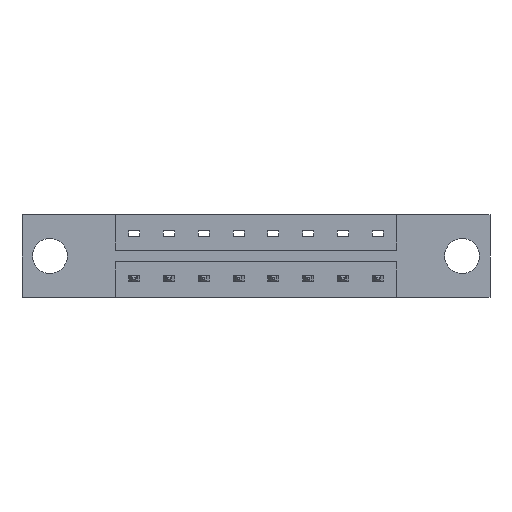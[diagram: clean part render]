
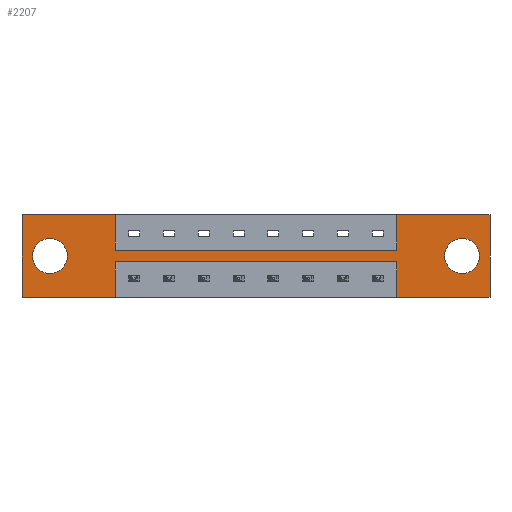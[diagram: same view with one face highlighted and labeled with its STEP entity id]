
A CAD part, front view. The second image highlights one B-rep face of the part: STEP entity #2207.
In plain terms, the highlighted planar face has unit normal (0, -1, 0).
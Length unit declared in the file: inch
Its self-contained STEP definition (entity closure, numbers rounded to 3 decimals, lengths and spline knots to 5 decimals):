
#139 = CARTESIAN_POINT ( 'NONE',  ( 0.125, 0., -0.107 ) ) ;
#160 = DIRECTION ( 'NONE',  ( 0., 1., 0. ) ) ;
#165 = CARTESIAN_POINT ( 'NONE',  ( 1.6785, 0., 0. ) ) ;
#324 = VERTEX_POINT ( 'NONE', #4264 ) ;
#367 = EDGE_CURVE ( 'NONE', #1852, #6719, #958, .T. ) ;
#611 = AXIS2_PLACEMENT_3D ( 'NONE', #2111, #160, #5095 ) ;
#616 = VECTOR ( 'NONE', #8769, 39.37008 ) ;
#666 = AXIS2_PLACEMENT_3D ( 'NONE', #2373, #1766, #8126 ) ;
#777 = CARTESIAN_POINT ( 'NONE',  ( 0., 0., 0. ) ) ;
#881 = ORIENTED_EDGE ( 'NONE', *, *, #7496, .F. ) ;
#884 = ORIENTED_EDGE ( 'NONE', *, *, #993, .F. ) ;
#929 = DIRECTION ( 'NONE',  ( -1., 0., 0. ) ) ;
#958 = LINE ( 'NONE', #1701, #5519 ) ;
#993 = EDGE_CURVE ( 'NONE', #8271, #3532, #1184, .T. ) ;
#1001 = DIRECTION ( 'NONE',  ( 1., 0., 0. ) ) ;
#1050 = CIRCLE ( 'NONE', #7961, 0.078 ) ;
#1163 = DIRECTION ( 'NONE',  ( 0., 0., -1. ) ) ;
#1184 = LINE ( 'NONE', #4027, #3704 ) ;
#1374 = ORIENTED_EDGE ( 'NONE', *, *, #8240, .F. ) ;
#1465 = DIRECTION ( 'NONE',  ( 0., 0., -1. ) ) ;
#1591 = CARTESIAN_POINT ( 'NONE',  ( 0.125, 0., -0.263 ) ) ;
#1646 = CARTESIAN_POINT ( 'NONE',  ( 0.4175, 0., 0. ) ) ;
#1683 = ORIENTED_EDGE ( 'NONE', *, *, #1780, .T. ) ;
#1701 = CARTESIAN_POINT ( 'NONE',  ( 1.6785, 0., -0.1585 ) ) ;
#1766 = DIRECTION ( 'NONE',  ( 0., 1., 0. ) ) ;
#1780 = EDGE_CURVE ( 'NONE', #3923, #2492, #1050, .T. ) ;
#1852 = VERTEX_POINT ( 'NONE', #2657 ) ;
#2101 = VECTOR ( 'NONE', #7195, 39.37008 ) ;
#2111 = CARTESIAN_POINT ( 'NONE',  ( 1.971, 0., -0.185 ) ) ;
#2207 = ADVANCED_FACE ( 'NONE', ( #9029, #5955, #2548 ), #5431, .T. ) ;
#2288 = CARTESIAN_POINT ( 'NONE',  ( 0., 0., 0. ) ) ;
#2294 = DIRECTION ( 'NONE',  ( 0., 0., 1. ) ) ;
#2360 = EDGE_CURVE ( 'NONE', #2492, #3923, #5554, .T. ) ;
#2368 = CARTESIAN_POINT ( 'NONE',  ( 0.125, 0., -0.185 ) ) ;
#2373 = CARTESIAN_POINT ( 'NONE',  ( 0.125, 0., -0.185 ) ) ;
#2471 = CARTESIAN_POINT ( 'NONE',  ( 1.971, 0., -0.185 ) ) ;
#2492 = VERTEX_POINT ( 'NONE', #3578 ) ;
#2548 = FACE_OUTER_BOUND ( 'NONE', #8283, .T. ) ;
#2581 = VECTOR ( 'NONE', #4423, 39.37008 ) ;
#2657 = CARTESIAN_POINT ( 'NONE',  ( 1.6785, 0., -0.1585 ) ) ;
#2668 = CARTESIAN_POINT ( 'NONE',  ( 1.6785, 0., -0.37 ) ) ;
#2714 = ORIENTED_EDGE ( 'NONE', *, *, #3780, .F. ) ;
#2778 = EDGE_CURVE ( 'NONE', #7587, #2853, #3658, .T. ) ;
#2853 = VERTEX_POINT ( 'NONE', #5265 ) ;
#2858 = VERTEX_POINT ( 'NONE', #139 ) ;
#3025 = CIRCLE ( 'NONE', #3169, 0.078 ) ;
#3159 = AXIS2_PLACEMENT_3D ( 'NONE', #8307, #8855, #7776 ) ;
#3169 = AXIS2_PLACEMENT_3D ( 'NONE', #2368, #5251, #8700 ) ;
#3174 = EDGE_CURVE ( 'NONE', #2858, #6212, #3025, .T. ) ;
#3183 = CARTESIAN_POINT ( 'NONE',  ( 0.4175, 0., -0.1585 ) ) ;
#3208 = DIRECTION ( 'NONE',  ( 0., 0., -1. ) ) ;
#3321 = EDGE_CURVE ( 'NONE', #2853, #8271, #4490, .T. ) ;
#3480 = VECTOR ( 'NONE', #1001, 39.37008 ) ;
#3532 = VERTEX_POINT ( 'NONE', #3537 ) ;
#3537 = CARTESIAN_POINT ( 'NONE',  ( 0.4175, 0., -0.1585 ) ) ;
#3578 = CARTESIAN_POINT ( 'NONE',  ( 1.971, 0., -0.107 ) ) ;
#3579 = CARTESIAN_POINT ( 'NONE',  ( 0.4175, 0., -0.2115 ) ) ;
#3658 = LINE ( 'NONE', #2288, #616 ) ;
#3704 = VECTOR ( 'NONE', #3208, 39.37008 ) ;
#3780 = EDGE_CURVE ( 'NONE', #6344, #8059, #5052, .T. ) ;
#3784 = ORIENTED_EDGE ( 'NONE', *, *, #6239, .T. ) ;
#3793 = LINE ( 'NONE', #4643, #6399 ) ;
#3923 = VERTEX_POINT ( 'NONE', #4716 ) ;
#4027 = CARTESIAN_POINT ( 'NONE',  ( 0.4175, 0., -0.1585 ) ) ;
#4037 = ORIENTED_EDGE ( 'NONE', *, *, #8281, .F. ) ;
#4127 = EDGE_CURVE ( 'NONE', #8059, #7587, #8682, .T. ) ;
#4264 = CARTESIAN_POINT ( 'NONE',  ( 1.6785, 0., -0.2115 ) ) ;
#4271 = CARTESIAN_POINT ( 'NONE',  ( 0., 0., -0.37 ) ) ;
#4311 = CARTESIAN_POINT ( 'NONE',  ( 2.096, 0., 0. ) ) ;
#4337 = EDGE_CURVE ( 'NONE', #6719, #4370, #6734, .T. ) ;
#4370 = VERTEX_POINT ( 'NONE', #5368 ) ;
#4417 = LINE ( 'NONE', #7296, #8925 ) ;
#4423 = DIRECTION ( 'NONE',  ( -1., 0., 0. ) ) ;
#4490 = LINE ( 'NONE', #777, #8286 ) ;
#4643 = CARTESIAN_POINT ( 'NONE',  ( 0.4175, 0., -0.2115 ) ) ;
#4656 = ORIENTED_EDGE ( 'NONE', *, *, #2778, .F. ) ;
#4716 = CARTESIAN_POINT ( 'NONE',  ( 1.971, 0., -0.263 ) ) ;
#4785 = ORIENTED_EDGE ( 'NONE', *, *, #7455, .F. ) ;
#5052 = LINE ( 'NONE', #3579, #7989 ) ;
#5095 = DIRECTION ( 'NONE',  ( 0., 0., -1. ) ) ;
#5203 = EDGE_LOOP ( 'NONE', ( #6758, #1683 ) ) ;
#5251 = DIRECTION ( 'NONE',  ( 0., 1., 0. ) ) ;
#5265 = CARTESIAN_POINT ( 'NONE',  ( 0., 0., 0. ) ) ;
#5368 = CARTESIAN_POINT ( 'NONE',  ( 2.096, 0., 0. ) ) ;
#5370 = EDGE_CURVE ( 'NONE', #8772, #8592, #8882, .T. ) ;
#5391 = DIRECTION ( 'NONE',  ( 1., 0., 0. ) ) ;
#5431 = PLANE ( 'NONE',  #3159 ) ;
#5436 = ORIENTED_EDGE ( 'NONE', *, *, #3174, .T. ) ;
#5519 = VECTOR ( 'NONE', #6508, 39.37008 ) ;
#5554 = CIRCLE ( 'NONE', #611, 0.078 ) ;
#5911 = VECTOR ( 'NONE', #8155, 39.37008 ) ;
#5955 = FACE_BOUND ( 'NONE', #8947, .T. ) ;
#5999 = CARTESIAN_POINT ( 'NONE',  ( 0., 0., -0.37 ) ) ;
#6203 = ORIENTED_EDGE ( 'NONE', *, *, #4127, .F. ) ;
#6212 = VERTEX_POINT ( 'NONE', #1591 ) ;
#6239 = EDGE_CURVE ( 'NONE', #6212, #2858, #8642, .T. ) ;
#6275 = CARTESIAN_POINT ( 'NONE',  ( 0.4175, 0., -0.37 ) ) ;
#6344 = VERTEX_POINT ( 'NONE', #7643 ) ;
#6399 = VECTOR ( 'NONE', #929, 39.37008 ) ;
#6508 = DIRECTION ( 'NONE',  ( 0., 0., 1. ) ) ;
#6719 = VERTEX_POINT ( 'NONE', #165 ) ;
#6734 = LINE ( 'NONE', #7398, #3480 ) ;
#6758 = ORIENTED_EDGE ( 'NONE', *, *, #2360, .T. ) ;
#7195 = DIRECTION ( 'NONE',  ( 0., 0., -1. ) ) ;
#7238 = ORIENTED_EDGE ( 'NONE', *, *, #5370, .F. ) ;
#7243 = ORIENTED_EDGE ( 'NONE', *, *, #3321, .F. ) ;
#7292 = VECTOR ( 'NONE', #5391, 39.37008 ) ;
#7296 = CARTESIAN_POINT ( 'NONE',  ( 1.6785, 0., -0.2115 ) ) ;
#7363 = ORIENTED_EDGE ( 'NONE', *, *, #4337, .F. ) ;
#7368 = DIRECTION ( 'NONE',  ( 1., 0., 0. ) ) ;
#7389 = LINE ( 'NONE', #4311, #2101 ) ;
#7398 = CARTESIAN_POINT ( 'NONE',  ( 0., 0., 0. ) ) ;
#7455 = EDGE_CURVE ( 'NONE', #3532, #1852, #8035, .T. ) ;
#7496 = EDGE_CURVE ( 'NONE', #324, #6344, #3793, .T. ) ;
#7587 = VERTEX_POINT ( 'NONE', #5999 ) ;
#7643 = CARTESIAN_POINT ( 'NONE',  ( 0.4175, 0., -0.2115 ) ) ;
#7776 = DIRECTION ( 'NONE',  ( 0., 0., -1. ) ) ;
#7961 = AXIS2_PLACEMENT_3D ( 'NONE', #2471, #8225, #1163 ) ;
#7989 = VECTOR ( 'NONE', #1465, 39.37008 ) ;
#8035 = LINE ( 'NONE', #3183, #7292 ) ;
#8059 = VERTEX_POINT ( 'NONE', #6275 ) ;
#8126 = DIRECTION ( 'NONE',  ( 0., 0., 1. ) ) ;
#8155 = DIRECTION ( 'NONE',  ( -1., 0., 0. ) ) ;
#8225 = DIRECTION ( 'NONE',  ( 0., 1., 0. ) ) ;
#8240 = EDGE_CURVE ( 'NONE', #8592, #324, #4417, .T. ) ;
#8271 = VERTEX_POINT ( 'NONE', #1646 ) ;
#8281 = EDGE_CURVE ( 'NONE', #4370, #8772, #7389, .T. ) ;
#8283 = EDGE_LOOP ( 'NONE', ( #1374, #7238, #4037, #7363, #8512, #4785, #884, #7243, #4656, #6203, #2714, #881 ) ) ;
#8285 = CARTESIAN_POINT ( 'NONE',  ( 0., 0., -0.37 ) ) ;
#8286 = VECTOR ( 'NONE', #7368, 39.37008 ) ;
#8307 = CARTESIAN_POINT ( 'NONE',  ( 0., 0., -0.37 ) ) ;
#8512 = ORIENTED_EDGE ( 'NONE', *, *, #367, .F. ) ;
#8592 = VERTEX_POINT ( 'NONE', #2668 ) ;
#8642 = CIRCLE ( 'NONE', #666, 0.078 ) ;
#8682 = LINE ( 'NONE', #4271, #2581 ) ;
#8700 = DIRECTION ( 'NONE',  ( 0., 0., 1. ) ) ;
#8769 = DIRECTION ( 'NONE',  ( 0., 0., 1. ) ) ;
#8772 = VERTEX_POINT ( 'NONE', #9249 ) ;
#8855 = DIRECTION ( 'NONE',  ( 0., -1., 0. ) ) ;
#8882 = LINE ( 'NONE', #8285, #5911 ) ;
#8925 = VECTOR ( 'NONE', #2294, 39.37008 ) ;
#8947 = EDGE_LOOP ( 'NONE', ( #5436, #3784 ) ) ;
#9029 = FACE_BOUND ( 'NONE', #5203, .T. ) ;
#9249 = CARTESIAN_POINT ( 'NONE',  ( 2.096, 0., -0.37 ) ) ;
